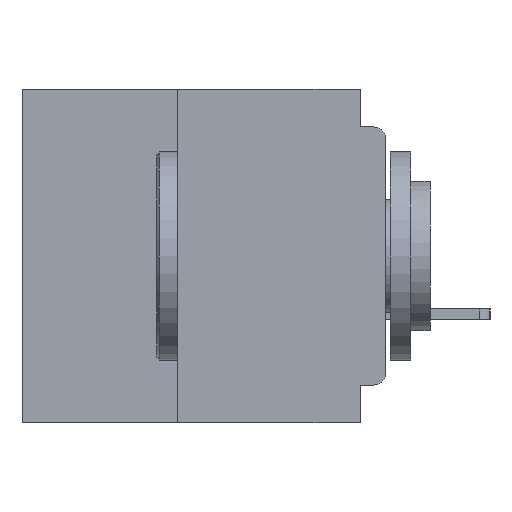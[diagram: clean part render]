
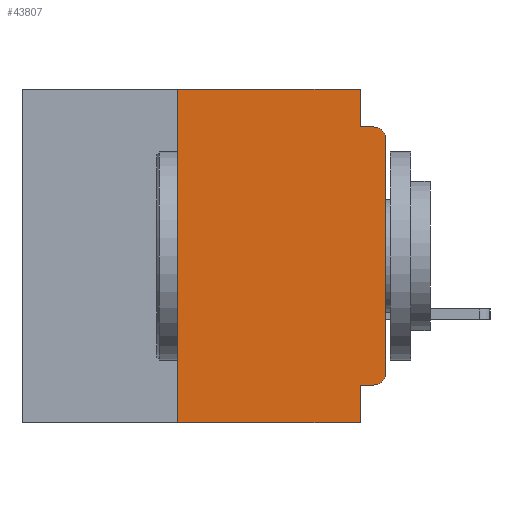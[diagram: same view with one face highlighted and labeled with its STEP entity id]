
A CAD part, left-side view. The second image highlights one B-rep face of the part: STEP entity #43807.
In plain terms, the highlighted planar face has unit normal (-1, 0, 0).
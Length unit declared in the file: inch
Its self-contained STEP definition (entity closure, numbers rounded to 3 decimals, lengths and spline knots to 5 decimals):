
#657 = ORIENTED_EDGE ( 'NONE', *, *, #22861, .T. ) ;
#853 = VERTEX_POINT ( 'NONE', #25060 ) ;
#1453 = DIRECTION ( 'NONE',  ( 0., 0., -1. ) ) ;
#2967 = VERTEX_POINT ( 'NONE', #26585 ) ;
#3315 = AXIS2_PLACEMENT_3D ( 'NONE', #21628, #48946, #25577 ) ;
#3567 = CARTESIAN_POINT ( 'NONE',  ( 0., 0.031, 0. ) ) ;
#3986 = VECTOR ( 'NONE', #6647, 39.37008 ) ;
#5002 = VERTEX_POINT ( 'NONE', #47572 ) ;
#6647 = DIRECTION ( 'NONE',  ( 0., 1., 0. ) ) ;
#6958 = DIRECTION ( 'NONE',  ( 0., 0., 1. ) ) ;
#8258 = ORIENTED_EDGE ( 'NONE', *, *, #47440, .F. ) ;
#8718 = LINE ( 'NONE', #45843, #28247 ) ;
#9557 = CARTESIAN_POINT ( 'NONE',  ( 0., 0.437, 0. ) ) ;
#10733 = CARTESIAN_POINT ( 'NONE',  ( 0., 0.015, -0.355 ) ) ;
#10976 = ORIENTED_EDGE ( 'NONE', *, *, #25738, .F. ) ;
#11417 = FACE_OUTER_BOUND ( 'NONE', #44106, .T. ) ;
#11520 = EDGE_CURVE ( 'NONE', #48908, #40957, #35809, .T. ) ;
#12312 = VECTOR ( 'NONE', #18616, 39.37008 ) ;
#13016 = CARTESIAN_POINT ( 'NONE',  ( 0., 0.031, -0.4 ) ) ;
#13318 = CARTESIAN_POINT ( 'NONE',  ( 0., 0.015, -0.06 ) ) ;
#13480 = DIRECTION ( 'NONE',  ( 0., 0., -1. ) ) ;
#13728 = LINE ( 'NONE', #13016, #22883 ) ;
#13943 = DIRECTION ( 'NONE',  ( 0., -1., 0. ) ) ;
#16281 = CARTESIAN_POINT ( 'NONE',  ( 0., 0.25, 0. ) ) ;
#16577 = VECTOR ( 'NONE', #24791, 39.37008 ) ;
#17210 = DIRECTION ( 'NONE',  ( 0., 0., -1. ) ) ;
#17269 = CARTESIAN_POINT ( 'NONE',  ( 0., 0.437, -0.4 ) ) ;
#17812 = CARTESIAN_POINT ( 'NONE',  ( 0., 0.437, 0. ) ) ;
#18616 = DIRECTION ( 'NONE',  ( 0., -1., 0. ) ) ;
#18683 = CARTESIAN_POINT ( 'NONE',  ( 0., 0.25, -0.4 ) ) ;
#19365 = CIRCLE ( 'NONE', #3315, 0.015 ) ;
#20212 = CARTESIAN_POINT ( 'NONE',  ( 0., 0., -0.06 ) ) ;
#21628 = CARTESIAN_POINT ( 'NONE',  ( 0., 0.015, -0.34 ) ) ;
#22298 = CARTESIAN_POINT ( 'NONE',  ( 0., 0., -0.355 ) ) ;
#22861 = EDGE_CURVE ( 'NONE', #32146, #48908, #8718, .T. ) ;
#22883 = VECTOR ( 'NONE', #1453, 39.37008 ) ;
#23520 = ORIENTED_EDGE ( 'NONE', *, *, #43418, .T. ) ;
#24134 = VERTEX_POINT ( 'NONE', #16281 ) ;
#24293 = EDGE_CURVE ( 'NONE', #48632, #853, #46842, .T. ) ;
#24726 = ORIENTED_EDGE ( 'NONE', *, *, #25601, .F. ) ;
#24791 = DIRECTION ( 'NONE',  ( 0., 0., 1. ) ) ;
#25060 = CARTESIAN_POINT ( 'NONE',  ( 0., 0.031, -0.4 ) ) ;
#25076 = PLANE ( 'NONE',  #46784 ) ;
#25577 = DIRECTION ( 'NONE',  ( 0., 0., -1. ) ) ;
#25601 = EDGE_CURVE ( 'NONE', #44017, #2967, #32639, .T. ) ;
#25738 = EDGE_CURVE ( 'NONE', #5002, #26927, #27747, .T. ) ;
#25767 = ORIENTED_EDGE ( 'NONE', *, *, #11520, .T. ) ;
#26555 = VECTOR ( 'NONE', #42591, 39.37008 ) ;
#26585 = CARTESIAN_POINT ( 'NONE',  ( 0., 0.031, -0.355 ) ) ;
#26927 = VERTEX_POINT ( 'NONE', #43679 ) ;
#27747 = LINE ( 'NONE', #3567, #26555 ) ;
#28247 = VECTOR ( 'NONE', #6958, 39.37008 ) ;
#29905 = VECTOR ( 'NONE', #13943, 39.37008 ) ;
#31559 = VECTOR ( 'NONE', #48534, 39.37008 ) ;
#32146 = VERTEX_POINT ( 'NONE', #42446 ) ;
#32639 = LINE ( 'NONE', #22298, #3986 ) ;
#34077 = ORIENTED_EDGE ( 'NONE', *, *, #45012, .F. ) ;
#34236 = EDGE_CURVE ( 'NONE', #24134, #5002, #40266, .T. ) ;
#34302 = ORIENTED_EDGE ( 'NONE', *, *, #24293, .T. ) ;
#34311 = LINE ( 'NONE', #45979, #12312 ) ;
#35809 = CIRCLE ( 'NONE', #36477, 0.015 ) ;
#36477 = AXIS2_PLACEMENT_3D ( 'NONE', #13318, #40634, #17210 ) ;
#36734 = CARTESIAN_POINT ( 'NONE',  ( 0., 0.015, -0.045 ) ) ;
#36862 = DIRECTION ( 'NONE',  ( 1., 0., 0. ) ) ;
#37370 = LINE ( 'NONE', #40330, #16577 ) ;
#37914 = EDGE_CURVE ( 'NONE', #48632, #24134, #37370, .T. ) ;
#40266 = LINE ( 'NONE', #17812, #29905 ) ;
#40330 = CARTESIAN_POINT ( 'NONE',  ( 0., 0.25, -0.4 ) ) ;
#40634 = DIRECTION ( 'NONE',  ( -1., 0., 0. ) ) ;
#40957 = VERTEX_POINT ( 'NONE', #36734 ) ;
#42446 = CARTESIAN_POINT ( 'NONE',  ( 0., 0., -0.34 ) ) ;
#42591 = DIRECTION ( 'NONE',  ( 0., 0., -1. ) ) ;
#43418 = EDGE_CURVE ( 'NONE', #44017, #32146, #19365, .T. ) ;
#43679 = CARTESIAN_POINT ( 'NONE',  ( 0., 0.031, -0.045 ) ) ;
#43807 = ADVANCED_FACE ( 'NONE', ( #11417 ), #25076, .F. ) ;
#44017 = VERTEX_POINT ( 'NONE', #10733 ) ;
#44106 = EDGE_LOOP ( 'NONE', ( #657, #25767, #8258, #10976, #47121, #45256, #34302, #34077, #24726, #23520 ) ) ;
#45012 = EDGE_CURVE ( 'NONE', #2967, #853, #13728, .T. ) ;
#45256 = ORIENTED_EDGE ( 'NONE', *, *, #37914, .F. ) ;
#45843 = CARTESIAN_POINT ( 'NONE',  ( 0., 0., 0. ) ) ;
#45979 = CARTESIAN_POINT ( 'NONE',  ( 0., 0., -0.045 ) ) ;
#46784 = AXIS2_PLACEMENT_3D ( 'NONE', #9557, #36862, #13480 ) ;
#46842 = LINE ( 'NONE', #17269, #31559 ) ;
#47121 = ORIENTED_EDGE ( 'NONE', *, *, #34236, .F. ) ;
#47440 = EDGE_CURVE ( 'NONE', #26927, #40957, #34311, .T. ) ;
#47572 = CARTESIAN_POINT ( 'NONE',  ( 0., 0.031, 0. ) ) ;
#48534 = DIRECTION ( 'NONE',  ( 0., -1., 0. ) ) ;
#48632 = VERTEX_POINT ( 'NONE', #18683 ) ;
#48908 = VERTEX_POINT ( 'NONE', #20212 ) ;
#48946 = DIRECTION ( 'NONE',  ( -1., 0., 0. ) ) ;
